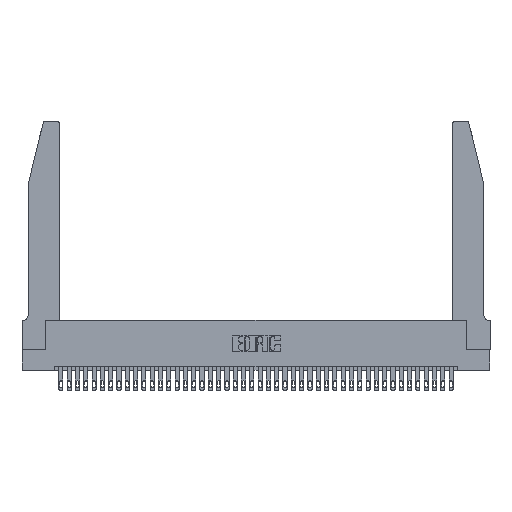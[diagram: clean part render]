
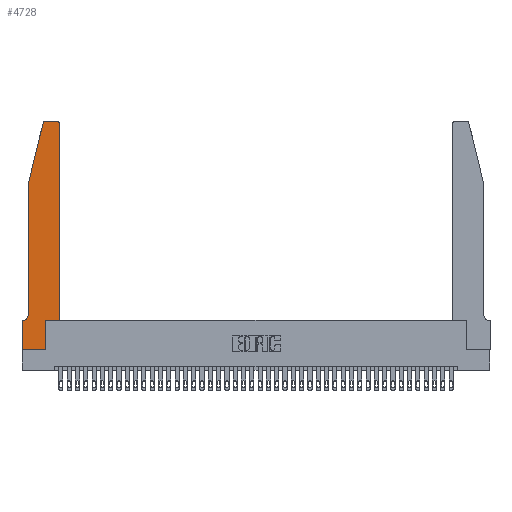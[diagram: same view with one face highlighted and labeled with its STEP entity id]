
A CAD part, top view. The second image highlights one B-rep face of the part: STEP entity #4728.
In plain terms, the highlighted planar face has unit normal (0, 0, 1).
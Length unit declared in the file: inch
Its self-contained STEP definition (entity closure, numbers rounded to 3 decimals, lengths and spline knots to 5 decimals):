
#184 = EDGE_LOOP ( 'NONE', ( #17982, #12835, #15218, #31328, #20570, #5142, #38763, #3699, #20090, #13304, #8216, #28405 ) ) ;
#551 = CARTESIAN_POINT ( 'NONE',  ( 0.0755, 0.35, 0.37 ) ) ;
#701 = CARTESIAN_POINT ( 'NONE',  ( 0., 0.35, 0.37 ) ) ;
#712 = VERTEX_POINT ( 'NONE', #25022 ) ;
#1796 = VECTOR ( 'NONE', #12050, 39.37008 ) ;
#1883 = AXIS2_PLACEMENT_3D ( 'NONE', #29213, #3636, #13795 ) ;
#1903 = EDGE_CURVE ( 'NONE', #8903, #13238, #10451, .T. ) ;
#2366 = DIRECTION ( 'NONE',  ( 0., -1., 0. ) ) ;
#3419 = DIRECTION ( 'NONE',  ( 0., -1., 0. ) ) ;
#3636 = DIRECTION ( 'NONE',  ( 0., 0., -1. ) ) ;
#3699 = ORIENTED_EDGE ( 'NONE', *, *, #19082, .T. ) ;
#4728 = ADVANCED_FACE ( 'NONE', ( #23538 ), #23081, .T. ) ;
#5142 = ORIENTED_EDGE ( 'NONE', *, *, #32974, .T. ) ;
#5178 = DIRECTION ( 'NONE',  ( 0., 1., 0. ) ) ;
#5642 = CIRCLE ( 'NONE', #40281, 0.03 ) ;
#5909 = LINE ( 'NONE', #8609, #40985 ) ;
#5990 = VERTEX_POINT ( 'NONE', #7486 ) ;
#6001 = EDGE_CURVE ( 'NONE', #8474, #11857, #5909, .T. ) ;
#6245 = EDGE_CURVE ( 'NONE', #18529, #35986, #19516, .T. ) ;
#7000 = EDGE_CURVE ( 'NONE', #5990, #18529, #7356, .T. ) ;
#7356 = LINE ( 'NONE', #28136, #1796 ) ;
#7486 = CARTESIAN_POINT ( 'NONE',  ( 0.25487, 2.72718, 0.37 ) ) ;
#7624 = DIRECTION ( 'NONE',  ( 0., 0., 1. ) ) ;
#7707 = VERTEX_POINT ( 'NONE', #27942 ) ;
#8095 = VECTOR ( 'NONE', #10899, 39.37008 ) ;
#8216 = ORIENTED_EDGE ( 'NONE', *, *, #6001, .T. ) ;
#8290 = CIRCLE ( 'NONE', #16053, 0.03 ) ;
#8474 = VERTEX_POINT ( 'NONE', #33982 ) ;
#8555 = VECTOR ( 'NONE', #37823, 39.37008 ) ;
#8609 = CARTESIAN_POINT ( 'NONE',  ( 0.4505, 0.35, 0.37 ) ) ;
#8654 = DIRECTION ( 'NONE',  ( -1., 0., 0. ) ) ;
#8903 = VERTEX_POINT ( 'NONE', #16638 ) ;
#9428 = CARTESIAN_POINT ( 'NONE',  ( 0., 0., 0.37 ) ) ;
#10451 = LINE ( 'NONE', #30634, #24009 ) ;
#10899 = DIRECTION ( 'NONE',  ( 0., 1., 0. ) ) ;
#11656 = EDGE_CURVE ( 'NONE', #35986, #712, #20975, .T. ) ;
#11724 = CARTESIAN_POINT ( 'NONE',  ( 0.4505, 0.35, 0.37 ) ) ;
#11857 = VERTEX_POINT ( 'NONE', #33104 ) ;
#11953 = CARTESIAN_POINT ( 'NONE',  ( 0., 0., 0.37 ) ) ;
#12050 = DIRECTION ( 'NONE',  ( -0.239, -0.971, 0. ) ) ;
#12835 = ORIENTED_EDGE ( 'NONE', *, *, #32862, .T. ) ;
#13238 = VERTEX_POINT ( 'NONE', #28391 ) ;
#13304 = ORIENTED_EDGE ( 'NONE', *, *, #36148, .T. ) ;
#13795 = DIRECTION ( 'NONE',  ( -1., 0., 0. ) ) ;
#14092 = LINE ( 'NONE', #11724, #8555 ) ;
#15218 = ORIENTED_EDGE ( 'NONE', *, *, #7000, .T. ) ;
#15305 = LINE ( 'NONE', #32197, #26319 ) ;
#15398 = EDGE_CURVE ( 'NONE', #11857, #8903, #8290, .T. ) ;
#16053 = AXIS2_PLACEMENT_3D ( 'NONE', #36323, #7624, #20428 ) ;
#16542 = VERTEX_POINT ( 'NONE', #23420 ) ;
#16638 = CARTESIAN_POINT ( 'NONE',  ( 0.4205, 2.75, 0.37 ) ) ;
#16664 = LINE ( 'NONE', #27131, #8095 ) ;
#17982 = ORIENTED_EDGE ( 'NONE', *, *, #1903, .T. ) ;
#18107 = VERTEX_POINT ( 'NONE', #9428 ) ;
#18529 = VERTEX_POINT ( 'NONE', #37110 ) ;
#18999 = CARTESIAN_POINT ( 'NONE',  ( 0.0755, 2., 0.37 ) ) ;
#19082 = EDGE_CURVE ( 'NONE', #18107, #23433, #39508, .T. ) ;
#19516 = LINE ( 'NONE', #18999, #29491 ) ;
#19647 = AXIS2_PLACEMENT_3D ( 'NONE', #701, #23214, #35660 ) ;
#20090 = ORIENTED_EDGE ( 'NONE', *, *, #27712, .T. ) ;
#20428 = DIRECTION ( 'NONE',  ( 1., 0., 0. ) ) ;
#20570 = ORIENTED_EDGE ( 'NONE', *, *, #11656, .T. ) ;
#20975 = CIRCLE ( 'NONE', #1883, 0.07 ) ;
#22366 = EDGE_CURVE ( 'NONE', #16542, #18107, #15305, .T. ) ;
#23081 = PLANE ( 'NONE',  #19647 ) ;
#23214 = DIRECTION ( 'NONE',  ( 0., 0., 1. ) ) ;
#23420 = CARTESIAN_POINT ( 'NONE',  ( 0., 0.35, 0.37 ) ) ;
#23433 = VERTEX_POINT ( 'NONE', #41471 ) ;
#23538 = FACE_OUTER_BOUND ( 'NONE', #184, .T. ) ;
#24009 = VECTOR ( 'NONE', #8654, 39.37008 ) ;
#24697 = DIRECTION ( 'NONE',  ( 1., 0., 0. ) ) ;
#25022 = CARTESIAN_POINT ( 'NONE',  ( 0.0055, 0.35, 0.37 ) ) ;
#26319 = VECTOR ( 'NONE', #3419, 39.37008 ) ;
#27131 = CARTESIAN_POINT ( 'NONE',  ( 0.2865, 0.35, 0.37 ) ) ;
#27260 = LINE ( 'NONE', #551, #40232 ) ;
#27712 = EDGE_CURVE ( 'NONE', #23433, #7707, #16664, .T. ) ;
#27942 = CARTESIAN_POINT ( 'NONE',  ( 0.2865, 0.35, 0.37 ) ) ;
#28136 = CARTESIAN_POINT ( 'NONE',  ( 0.0755, 2., 0.37 ) ) ;
#28391 = CARTESIAN_POINT ( 'NONE',  ( 0.284, 2.75, 0.37 ) ) ;
#28405 = ORIENTED_EDGE ( 'NONE', *, *, #15398, .T. ) ;
#29213 = CARTESIAN_POINT ( 'NONE',  ( 0.0055, 0.42, 0.37 ) ) ;
#29491 = VECTOR ( 'NONE', #2366, 39.37008 ) ;
#30521 = VECTOR ( 'NONE', #24697, 39.37008 ) ;
#30634 = CARTESIAN_POINT ( 'NONE',  ( 0.2605, 2.75, 0.37 ) ) ;
#31152 = DIRECTION ( 'NONE',  ( 1., 0., 0. ) ) ;
#31328 = ORIENTED_EDGE ( 'NONE', *, *, #6245, .T. ) ;
#32197 = CARTESIAN_POINT ( 'NONE',  ( 0., 0., 0.37 ) ) ;
#32862 = EDGE_CURVE ( 'NONE', #13238, #5990, #5642, .T. ) ;
#32974 = EDGE_CURVE ( 'NONE', #712, #16542, #27260, .T. ) ;
#33104 = CARTESIAN_POINT ( 'NONE',  ( 0.4505, 2.72, 0.37 ) ) ;
#33416 = CARTESIAN_POINT ( 'NONE',  ( 0.0755, 0.42, 0.37 ) ) ;
#33982 = CARTESIAN_POINT ( 'NONE',  ( 0.4505, 0.35, 0.37 ) ) ;
#35660 = DIRECTION ( 'NONE',  ( 1., 0., 0. ) ) ;
#35986 = VERTEX_POINT ( 'NONE', #33416 ) ;
#36148 = EDGE_CURVE ( 'NONE', #7707, #8474, #14092, .T. ) ;
#36323 = CARTESIAN_POINT ( 'NONE',  ( 0.4205, 2.72, 0.37 ) ) ;
#37110 = CARTESIAN_POINT ( 'NONE',  ( 0.0755, 2., 0.37 ) ) ;
#37434 = CARTESIAN_POINT ( 'NONE',  ( 0.284, 2.72, 0.37 ) ) ;
#37823 = DIRECTION ( 'NONE',  ( 1., 0., 0. ) ) ;
#38548 = DIRECTION ( 'NONE',  ( -1., 0., 0. ) ) ;
#38763 = ORIENTED_EDGE ( 'NONE', *, *, #22366, .T. ) ;
#39508 = LINE ( 'NONE', #11953, #30521 ) ;
#40232 = VECTOR ( 'NONE', #38548, 39.37008 ) ;
#40281 = AXIS2_PLACEMENT_3D ( 'NONE', #37434, #40362, #31152 ) ;
#40362 = DIRECTION ( 'NONE',  ( 0., 0., 1. ) ) ;
#40985 = VECTOR ( 'NONE', #5178, 39.37008 ) ;
#41471 = CARTESIAN_POINT ( 'NONE',  ( 0.2865, 0., 0.37 ) ) ;
